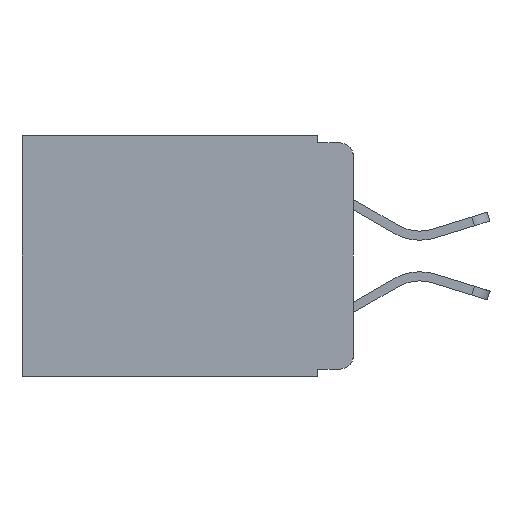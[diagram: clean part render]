
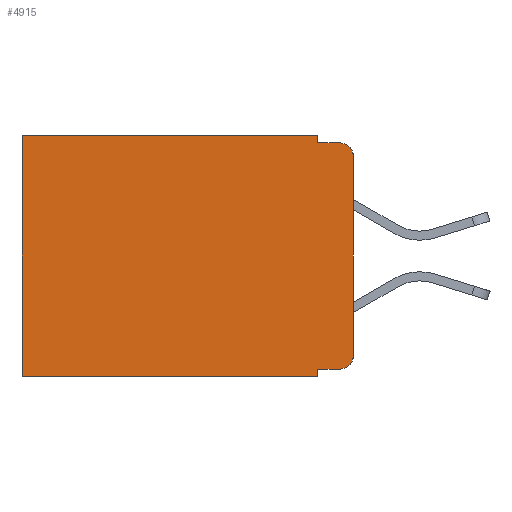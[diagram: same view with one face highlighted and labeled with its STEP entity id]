
A CAD part, left-side view. The second image highlights one B-rep face of the part: STEP entity #4915.
In plain terms, the highlighted planar face has unit normal (-1, 0, 0).
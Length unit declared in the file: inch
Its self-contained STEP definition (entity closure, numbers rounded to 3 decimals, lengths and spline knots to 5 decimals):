
#93 = DIRECTION ( 'NONE',  ( -1., 0., 0. ) ) ;
#254 = CARTESIAN_POINT ( 'NONE',  ( 0.298, 0., -0.03 ) ) ;
#370 = CARTESIAN_POINT ( 'NONE',  ( 0.298, 0.051, -0.01 ) ) ;
#615 = CARTESIAN_POINT ( 'NONE',  ( 0.298, 0.051, 0. ) ) ;
#787 = DIRECTION ( 'NONE',  ( 0., 0., -1. ) ) ;
#850 = VECTOR ( 'NONE', #4877, 39.37008 ) ;
#1000 = EDGE_CURVE ( 'NONE', #5351, #2627, #9793, .T. ) ;
#1108 = EDGE_CURVE ( 'NONE', #9192, #2627, #5045, .T. ) ;
#1111 = CARTESIAN_POINT ( 'NONE',  ( 0.298, 0.02, -0.01 ) ) ;
#1318 = LINE ( 'NONE', #615, #1939 ) ;
#1330 = LINE ( 'NONE', #2074, #3720 ) ;
#1939 = VECTOR ( 'NONE', #10981, 39.37008 ) ;
#2074 = CARTESIAN_POINT ( 'NONE',  ( 0.298, 0., 0. ) ) ;
#2226 = CARTESIAN_POINT ( 'NONE',  ( 0.298, 0.02, -0.03 ) ) ;
#2627 = VERTEX_POINT ( 'NONE', #1111 ) ;
#2641 = ORIENTED_EDGE ( 'NONE', *, *, #3790, .F. ) ;
#2660 = CARTESIAN_POINT ( 'NONE',  ( 0.298, 0.473, -0.343 ) ) ;
#2681 = CARTESIAN_POINT ( 'NONE',  ( 0.298, 0.473, 0. ) ) ;
#2918 = LINE ( 'NONE', #5048, #850 ) ;
#3179 = EDGE_CURVE ( 'NONE', #9192, #5627, #1330, .T. ) ;
#3349 = EDGE_CURVE ( 'NONE', #12009, #7076, #5493, .T. ) ;
#3436 = CARTESIAN_POINT ( 'NONE',  ( 0.298, 0.051, -0.01 ) ) ;
#3720 = VECTOR ( 'NONE', #9301, 39.37008 ) ;
#3790 = EDGE_CURVE ( 'NONE', #10543, #4072, #2918, .T. ) ;
#3843 = DIRECTION ( 'NONE',  ( 0., 0., -1. ) ) ;
#3847 = EDGE_CURVE ( 'NONE', #4253, #5627, #12747, .T. ) ;
#4072 = VERTEX_POINT ( 'NONE', #2660 ) ;
#4204 = VERTEX_POINT ( 'NONE', #9193 ) ;
#4211 = ORIENTED_EDGE ( 'NONE', *, *, #4713, .T. ) ;
#4251 = ORIENTED_EDGE ( 'NONE', *, *, #3179, .F. ) ;
#4253 = VERTEX_POINT ( 'NONE', #11316 ) ;
#4426 = CARTESIAN_POINT ( 'NONE',  ( 0.298, 0.051, 0. ) ) ;
#4527 = VECTOR ( 'NONE', #13340, 39.37008 ) ;
#4713 = EDGE_CURVE ( 'NONE', #4204, #4253, #7254, .T. ) ;
#4838 = EDGE_LOOP ( 'NONE', ( #4251, #12818, #7859, #7639, #6117, #12095, #2641, #6979, #4211, #10311 ) ) ;
#4842 = DIRECTION ( 'NONE',  ( 0., 0., -1. ) ) ;
#4877 = DIRECTION ( 'NONE',  ( 0., 1., 0. ) ) ;
#4915 = ADVANCED_FACE ( 'NONE', ( #8041 ), #11073, .F. ) ;
#5045 = CIRCLE ( 'NONE', #6024, 0.02 ) ;
#5048 = CARTESIAN_POINT ( 'NONE',  ( 0.298, 0., -0.343 ) ) ;
#5351 = VERTEX_POINT ( 'NONE', #3436 ) ;
#5493 = LINE ( 'NONE', #12292, #4527 ) ;
#5580 = EDGE_CURVE ( 'NONE', #12009, #5351, #6886, .T. ) ;
#5621 = CARTESIAN_POINT ( 'NONE',  ( 0.298, 0.051, -0.333 ) ) ;
#5627 = VERTEX_POINT ( 'NONE', #7271 ) ;
#5862 = CARTESIAN_POINT ( 'NONE',  ( 0.298, 0., 0. ) ) ;
#6024 = AXIS2_PLACEMENT_3D ( 'NONE', #2226, #12705, #7251 ) ;
#6117 = ORIENTED_EDGE ( 'NONE', *, *, #3349, .T. ) ;
#6190 = CARTESIAN_POINT ( 'NONE',  ( 0.298, 0.051, -0.343 ) ) ;
#6580 = VECTOR ( 'NONE', #3843, 39.37008 ) ;
#6886 = LINE ( 'NONE', #10086, #6580 ) ;
#6979 = ORIENTED_EDGE ( 'NONE', *, *, #12259, .F. ) ;
#7076 = VERTEX_POINT ( 'NONE', #2681 ) ;
#7211 = EDGE_CURVE ( 'NONE', #7076, #4072, #13263, .T. ) ;
#7251 = DIRECTION ( 'NONE',  ( 0., 0., -1. ) ) ;
#7254 = LINE ( 'NONE', #5621, #12189 ) ;
#7271 = CARTESIAN_POINT ( 'NONE',  ( 0.298, 0., -0.313 ) ) ;
#7639 = ORIENTED_EDGE ( 'NONE', *, *, #5580, .F. ) ;
#7859 = ORIENTED_EDGE ( 'NONE', *, *, #1000, .F. ) ;
#7893 = CARTESIAN_POINT ( 'NONE',  ( 0.298, 0.473, 0. ) ) ;
#8041 = FACE_OUTER_BOUND ( 'NONE', #4838, .T. ) ;
#8296 = DIRECTION ( 'NONE',  ( 0., 0., -1. ) ) ;
#8527 = AXIS2_PLACEMENT_3D ( 'NONE', #5862, #11165, #787 ) ;
#8596 = DIRECTION ( 'NONE',  ( 0., -1., 0. ) ) ;
#9192 = VERTEX_POINT ( 'NONE', #254 ) ;
#9193 = CARTESIAN_POINT ( 'NONE',  ( 0.298, 0.051, -0.333 ) ) ;
#9301 = DIRECTION ( 'NONE',  ( 0., 0., -1. ) ) ;
#9793 = LINE ( 'NONE', #370, #12444 ) ;
#9882 = AXIS2_PLACEMENT_3D ( 'NONE', #11513, #93, #8296 ) ;
#10086 = CARTESIAN_POINT ( 'NONE',  ( 0.298, 0.051, 0. ) ) ;
#10311 = ORIENTED_EDGE ( 'NONE', *, *, #3847, .T. ) ;
#10543 = VERTEX_POINT ( 'NONE', #6190 ) ;
#10981 = DIRECTION ( 'NONE',  ( 0., 0., -1. ) ) ;
#11073 = PLANE ( 'NONE',  #8527 ) ;
#11136 = VECTOR ( 'NONE', #4842, 39.37008 ) ;
#11165 = DIRECTION ( 'NONE',  ( 1., 0., 0. ) ) ;
#11316 = CARTESIAN_POINT ( 'NONE',  ( 0.298, 0.02, -0.333 ) ) ;
#11513 = CARTESIAN_POINT ( 'NONE',  ( 0.298, 0.02, -0.313 ) ) ;
#12009 = VERTEX_POINT ( 'NONE', #4426 ) ;
#12095 = ORIENTED_EDGE ( 'NONE', *, *, #7211, .T. ) ;
#12189 = VECTOR ( 'NONE', #13046, 39.37008 ) ;
#12259 = EDGE_CURVE ( 'NONE', #4204, #10543, #1318, .T. ) ;
#12292 = CARTESIAN_POINT ( 'NONE',  ( 0.298, 0., 0. ) ) ;
#12444 = VECTOR ( 'NONE', #8596, 39.37008 ) ;
#12705 = DIRECTION ( 'NONE',  ( -1., 0., 0. ) ) ;
#12747 = CIRCLE ( 'NONE', #9882, 0.02 ) ;
#12818 = ORIENTED_EDGE ( 'NONE', *, *, #1108, .T. ) ;
#13046 = DIRECTION ( 'NONE',  ( 0., -1., 0. ) ) ;
#13263 = LINE ( 'NONE', #7893, #11136 ) ;
#13340 = DIRECTION ( 'NONE',  ( 0., 1., 0. ) ) ;
